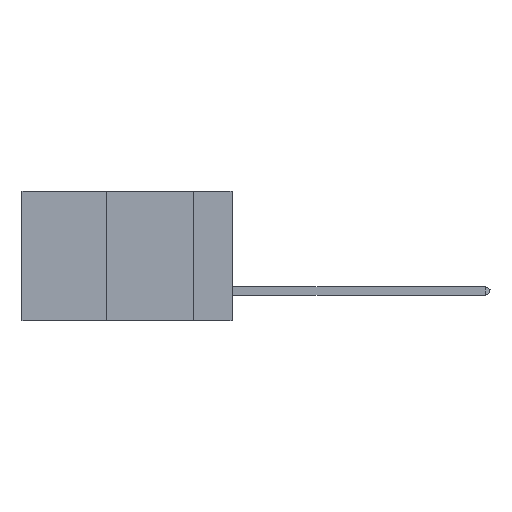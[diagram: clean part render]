
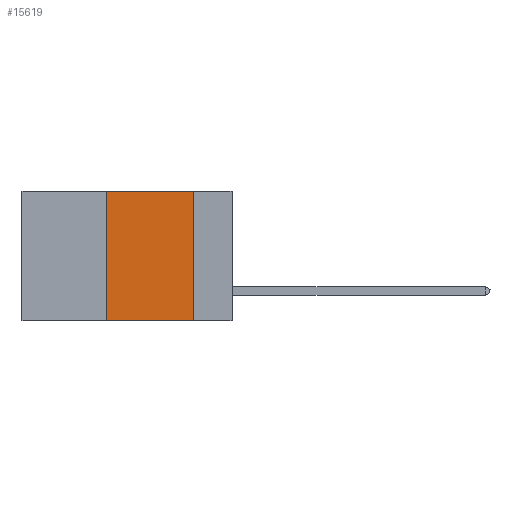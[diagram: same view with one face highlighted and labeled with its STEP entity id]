
A CAD part, left-side view. The second image highlights one B-rep face of the part: STEP entity #15619.
In plain terms, the highlighted planar face has unit normal (-1, 0, 0).
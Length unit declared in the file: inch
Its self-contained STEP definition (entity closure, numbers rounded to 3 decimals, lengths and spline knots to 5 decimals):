
#97 = DIRECTION ( 'NONE',  ( 1., 0., 0. ) ) ;
#613 = DIRECTION ( 'NONE',  ( 0., -1., 0. ) ) ;
#1604 = LINE ( 'NONE', #23623, #23772 ) ;
#2655 = ORIENTED_EDGE ( 'NONE', *, *, #26619, .F. ) ;
#2900 = DIRECTION ( 'NONE',  ( 0., -1., 0. ) ) ;
#3331 = EDGE_CURVE ( 'NONE', #21058, #23681, #21231, .T. ) ;
#3511 = DIRECTION ( 'NONE',  ( 0., 0., 1. ) ) ;
#4478 = EDGE_CURVE ( 'NONE', #21058, #18667, #14208, .T. ) ;
#5889 = CARTESIAN_POINT ( 'NONE',  ( 0., 0.36, 0. ) ) ;
#6242 = VECTOR ( 'NONE', #19527, 39.37008 ) ;
#7600 = VECTOR ( 'NONE', #2900, 39.37008 ) ;
#8269 = ORIENTED_EDGE ( 'NONE', *, *, #4478, .T. ) ;
#8363 = VECTOR ( 'NONE', #3511, 39.37008 ) ;
#8420 = CARTESIAN_POINT ( 'NONE',  ( 0., 0.36, 0. ) ) ;
#9615 = CARTESIAN_POINT ( 'NONE',  ( 0., 0.36, -0.37 ) ) ;
#10572 = VERTEX_POINT ( 'NONE', #22297 ) ;
#11839 = EDGE_LOOP ( 'NONE', ( #2655, #18013, #26764, #8269 ) ) ;
#11865 = LINE ( 'NONE', #19259, #6242 ) ;
#13110 = PLANE ( 'NONE',  #19487 ) ;
#14208 = LINE ( 'NONE', #19401, #7600 ) ;
#15230 = CARTESIAN_POINT ( 'NONE',  ( 0., 0.6, 0. ) ) ;
#15619 = ADVANCED_FACE ( 'NONE', ( #18624 ), #13110, .F. ) ;
#16988 = CARTESIAN_POINT ( 'NONE',  ( 0., 0.11, -0.37 ) ) ;
#18013 = ORIENTED_EDGE ( 'NONE', *, *, #26545, .F. ) ;
#18624 = FACE_OUTER_BOUND ( 'NONE', #11839, .T. ) ;
#18667 = VERTEX_POINT ( 'NONE', #16988 ) ;
#19259 = CARTESIAN_POINT ( 'NONE',  ( 0., 0.11, 0. ) ) ;
#19401 = CARTESIAN_POINT ( 'NONE',  ( 0., 0.6, -0.37 ) ) ;
#19487 = AXIS2_PLACEMENT_3D ( 'NONE', #15230, #97, #26282 ) ;
#19527 = DIRECTION ( 'NONE',  ( 0., 0., -1. ) ) ;
#21058 = VERTEX_POINT ( 'NONE', #9615 ) ;
#21231 = LINE ( 'NONE', #5889, #8363 ) ;
#22297 = CARTESIAN_POINT ( 'NONE',  ( 0., 0.11, 0. ) ) ;
#23623 = CARTESIAN_POINT ( 'NONE',  ( 0., 0.6, 0. ) ) ;
#23681 = VERTEX_POINT ( 'NONE', #8420 ) ;
#23772 = VECTOR ( 'NONE', #613, 39.37008 ) ;
#26282 = DIRECTION ( 'NONE',  ( 0., 0., -1. ) ) ;
#26545 = EDGE_CURVE ( 'NONE', #23681, #10572, #1604, .T. ) ;
#26619 = EDGE_CURVE ( 'NONE', #10572, #18667, #11865, .T. ) ;
#26764 = ORIENTED_EDGE ( 'NONE', *, *, #3331, .F. ) ;
